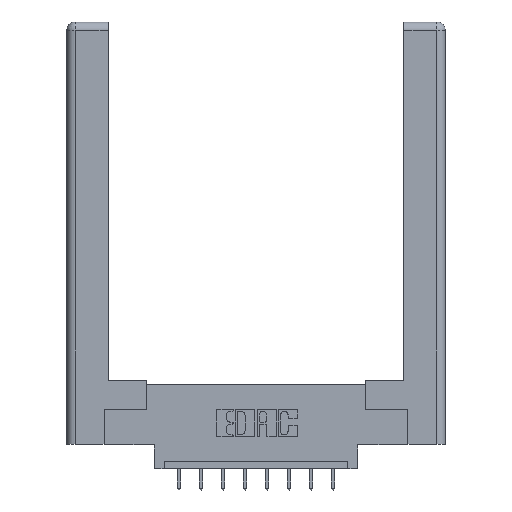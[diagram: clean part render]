
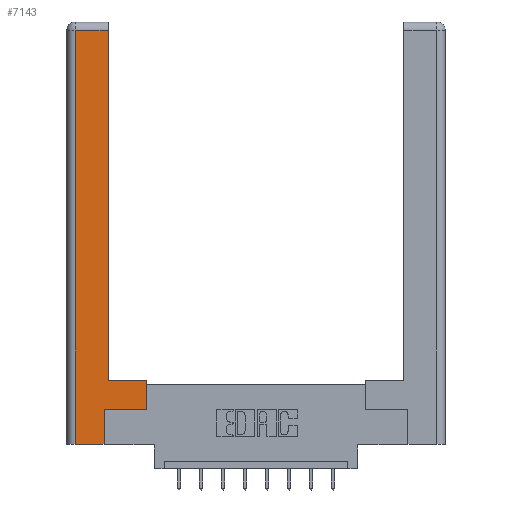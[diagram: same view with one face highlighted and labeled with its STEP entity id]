
A CAD part, top view. The second image highlights one B-rep face of the part: STEP entity #7143.
In plain terms, the highlighted planar face has unit normal (0, 0, 1).
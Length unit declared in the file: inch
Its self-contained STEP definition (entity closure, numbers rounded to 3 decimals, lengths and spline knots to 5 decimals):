
#481 = LINE ( 'NONE', #10847, #12540 ) ;
#606 = AXIS2_PLACEMENT_3D ( 'NONE', #12775, #9791, #2629 ) ;
#699 = CARTESIAN_POINT ( 'NONE',  ( 0.0615, 0., 0. ) ) ;
#705 = PLANE ( 'NONE',  #606 ) ;
#989 = EDGE_CURVE ( 'NONE', #9449, #2139, #10469, .T. ) ;
#1428 = ORIENTED_EDGE ( 'NONE', *, *, #3385, .T. ) ;
#1657 = CARTESIAN_POINT ( 'NONE',  ( 0.295, 2.94, 0. ) ) ;
#1684 = ORIENTED_EDGE ( 'NONE', *, *, #8857, .T. ) ;
#1708 = VERTEX_POINT ( 'NONE', #2523 ) ;
#2074 = VECTOR ( 'NONE', #8948, 39.37008 ) ;
#2139 = VERTEX_POINT ( 'NONE', #12852 ) ;
#2165 = ORIENTED_EDGE ( 'NONE', *, *, #989, .T. ) ;
#2398 = CARTESIAN_POINT ( 'NONE',  ( 0.295, 3., 0. ) ) ;
#2472 = VERTEX_POINT ( 'NONE', #11247 ) ;
#2523 = CARTESIAN_POINT ( 'NONE',  ( 0.565, 0.245, 0. ) ) ;
#2562 = CARTESIAN_POINT ( 'NONE',  ( 0.265, 0.245, 0. ) ) ;
#2629 = DIRECTION ( 'NONE',  ( -1., 0., 0. ) ) ;
#2751 = ORIENTED_EDGE ( 'NONE', *, *, #8011, .T. ) ;
#2943 = VERTEX_POINT ( 'NONE', #5607 ) ;
#2981 = VERTEX_POINT ( 'NONE', #1657 ) ;
#3099 = LINE ( 'NONE', #6724, #10877 ) ;
#3105 = VERTEX_POINT ( 'NONE', #12753 ) ;
#3274 = VECTOR ( 'NONE', #9503, 39.37008 ) ;
#3385 = EDGE_CURVE ( 'NONE', #2981, #3105, #4720, .T. ) ;
#3392 = DIRECTION ( 'NONE',  ( 0., 1., 0. ) ) ;
#3446 = DIRECTION ( 'NONE',  ( 0., -1., 0. ) ) ;
#3942 = ORIENTED_EDGE ( 'NONE', *, *, #8536, .T. ) ;
#3986 = LINE ( 'NONE', #2562, #5889 ) ;
#4037 = EDGE_CURVE ( 'NONE', #3105, #9449, #3099, .T. ) ;
#4287 = VECTOR ( 'NONE', #4300, 39.37008 ) ;
#4300 = DIRECTION ( 'NONE',  ( 1., 0., 0. ) ) ;
#4563 = EDGE_LOOP ( 'NONE', ( #6253, #1428, #8864, #2165, #2751, #3942, #6037, #1684 ) ) ;
#4720 = LINE ( 'NONE', #12019, #5183 ) ;
#5036 = DIRECTION ( 'NONE',  ( -1., 0., 0. ) ) ;
#5183 = VECTOR ( 'NONE', #5036, 39.37008 ) ;
#5607 = CARTESIAN_POINT ( 'NONE',  ( 0.265, 0.245, 0. ) ) ;
#5889 = VECTOR ( 'NONE', #6627, 39.37008 ) ;
#6037 = ORIENTED_EDGE ( 'NONE', *, *, #11818, .T. ) ;
#6253 = ORIENTED_EDGE ( 'NONE', *, *, #9710, .T. ) ;
#6627 = DIRECTION ( 'NONE',  ( 0., 1., 0. ) ) ;
#6724 = CARTESIAN_POINT ( 'NONE',  ( 0.0615, 0., 0. ) ) ;
#6769 = LINE ( 'NONE', #2398, #3274 ) ;
#7143 = ADVANCED_FACE ( 'NONE', ( #9238 ), #705, .F. ) ;
#7347 = CARTESIAN_POINT ( 'NONE',  ( 0.565, 0.45, 0. ) ) ;
#7971 = CARTESIAN_POINT ( 'NONE',  ( 0.565, 0.245, 0. ) ) ;
#8011 = EDGE_CURVE ( 'NONE', #2139, #2943, #3986, .T. ) ;
#8536 = EDGE_CURVE ( 'NONE', #2943, #1708, #11251, .T. ) ;
#8857 = EDGE_CURVE ( 'NONE', #11002, #2472, #481, .T. ) ;
#8864 = ORIENTED_EDGE ( 'NONE', *, *, #4037, .T. ) ;
#8948 = DIRECTION ( 'NONE',  ( 1., 0., 0. ) ) ;
#9238 = FACE_OUTER_BOUND ( 'NONE', #4563, .T. ) ;
#9343 = CARTESIAN_POINT ( 'NONE',  ( 0.265, 0., 0. ) ) ;
#9449 = VERTEX_POINT ( 'NONE', #699 ) ;
#9503 = DIRECTION ( 'NONE',  ( 0., 1., 0. ) ) ;
#9710 = EDGE_CURVE ( 'NONE', #2472, #2981, #6769, .T. ) ;
#9791 = DIRECTION ( 'NONE',  ( 0., 0., -1. ) ) ;
#9931 = DIRECTION ( 'NONE',  ( -1., 0., 0. ) ) ;
#10469 = LINE ( 'NONE', #9343, #4287 ) ;
#10715 = LINE ( 'NONE', #7347, #12452 ) ;
#10847 = CARTESIAN_POINT ( 'NONE',  ( 0.295, 0.45, 0. ) ) ;
#10877 = VECTOR ( 'NONE', #3446, 39.37008 ) ;
#11002 = VERTEX_POINT ( 'NONE', #12938 ) ;
#11247 = CARTESIAN_POINT ( 'NONE',  ( 0.295, 0.45, 0. ) ) ;
#11251 = LINE ( 'NONE', #7971, #2074 ) ;
#11818 = EDGE_CURVE ( 'NONE', #1708, #11002, #10715, .T. ) ;
#12019 = CARTESIAN_POINT ( 'NONE',  ( 0.0615, 2.94, 0. ) ) ;
#12452 = VECTOR ( 'NONE', #3392, 39.37008 ) ;
#12540 = VECTOR ( 'NONE', #9931, 39.37008 ) ;
#12753 = CARTESIAN_POINT ( 'NONE',  ( 0.0615, 2.94, 0. ) ) ;
#12775 = CARTESIAN_POINT ( 'NONE',  ( 0., 0., 0. ) ) ;
#12852 = CARTESIAN_POINT ( 'NONE',  ( 0.265, 0., 0. ) ) ;
#12938 = CARTESIAN_POINT ( 'NONE',  ( 0.565, 0.45, 0. ) ) ;
